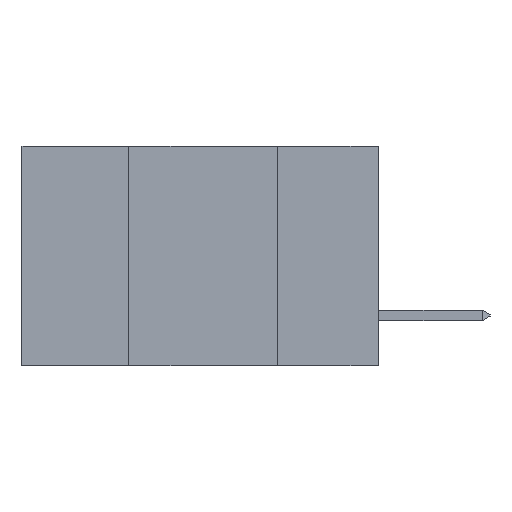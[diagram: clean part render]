
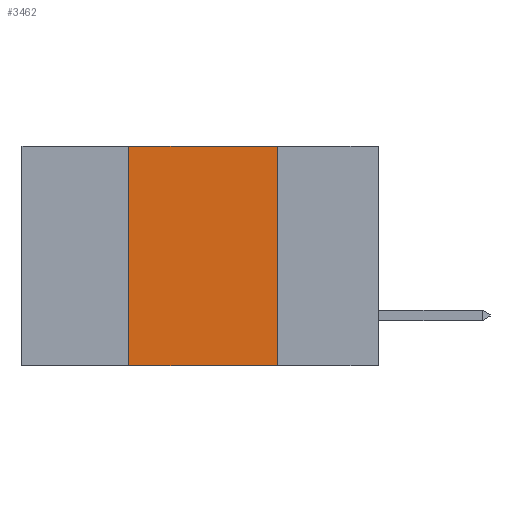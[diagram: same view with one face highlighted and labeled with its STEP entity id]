
A CAD part, left-side view. The second image highlights one B-rep face of the part: STEP entity #3462.
In plain terms, the highlighted planar face has unit normal (-1, 0, 0).
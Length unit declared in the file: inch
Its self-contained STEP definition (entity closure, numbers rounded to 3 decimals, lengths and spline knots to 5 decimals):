
#441 = LINE ( 'NONE', #831, #7234 ) ;
#478 = VERTEX_POINT ( 'NONE', #2760 ) ;
#831 = CARTESIAN_POINT ( 'NONE',  ( 0., 0.6, -0.37 ) ) ;
#945 = LINE ( 'NONE', #14482, #8116 ) ;
#1266 = VECTOR ( 'NONE', #4823, 39.37008 ) ;
#1758 = VECTOR ( 'NONE', #12450, 39.37008 ) ;
#2201 = CARTESIAN_POINT ( 'NONE',  ( 0., 0.42, -0.37 ) ) ;
#2386 = EDGE_CURVE ( 'NONE', #11320, #3335, #945, .T. ) ;
#2760 = CARTESIAN_POINT ( 'NONE',  ( 0., 0.17, -0.37 ) ) ;
#3335 = VERTEX_POINT ( 'NONE', #6868 ) ;
#3462 = ADVANCED_FACE ( 'NONE', ( #12043 ), #9267, .F. ) ;
#3794 = VERTEX_POINT ( 'NONE', #2201 ) ;
#4823 = DIRECTION ( 'NONE',  ( 0., 0., 1. ) ) ;
#6344 = ORIENTED_EDGE ( 'NONE', *, *, #2386, .F. ) ;
#6868 = CARTESIAN_POINT ( 'NONE',  ( 0., 0.17, 0. ) ) ;
#7234 = VECTOR ( 'NONE', #13904, 39.37008 ) ;
#8116 = VECTOR ( 'NONE', #15686, 39.37008 ) ;
#8191 = AXIS2_PLACEMENT_3D ( 'NONE', #12550, #12734, #11760 ) ;
#8666 = CARTESIAN_POINT ( 'NONE',  ( 0., 0.17, 0. ) ) ;
#9227 = LINE ( 'NONE', #8666, #1758 ) ;
#9267 = PLANE ( 'NONE',  #8191 ) ;
#10671 = EDGE_LOOP ( 'NONE', ( #13750, #6344, #16018, #13999 ) ) ;
#10737 = EDGE_CURVE ( 'NONE', #3335, #478, #9227, .T. ) ;
#10843 = EDGE_CURVE ( 'NONE', #3794, #478, #441, .T. ) ;
#11320 = VERTEX_POINT ( 'NONE', #14711 ) ;
#11691 = EDGE_CURVE ( 'NONE', #3794, #11320, #14331, .T. ) ;
#11760 = DIRECTION ( 'NONE',  ( 0., 0., -1. ) ) ;
#12043 = FACE_OUTER_BOUND ( 'NONE', #10671, .T. ) ;
#12450 = DIRECTION ( 'NONE',  ( 0., 0., -1. ) ) ;
#12550 = CARTESIAN_POINT ( 'NONE',  ( 0., 0.6, 0. ) ) ;
#12560 = CARTESIAN_POINT ( 'NONE',  ( 0., 0.42, 0. ) ) ;
#12734 = DIRECTION ( 'NONE',  ( 1., 0., 0. ) ) ;
#13750 = ORIENTED_EDGE ( 'NONE', *, *, #10737, .F. ) ;
#13904 = DIRECTION ( 'NONE',  ( 0., -1., 0. ) ) ;
#13999 = ORIENTED_EDGE ( 'NONE', *, *, #10843, .T. ) ;
#14331 = LINE ( 'NONE', #12560, #1266 ) ;
#14482 = CARTESIAN_POINT ( 'NONE',  ( 0., 0.6, 0. ) ) ;
#14711 = CARTESIAN_POINT ( 'NONE',  ( 0., 0.42, 0. ) ) ;
#15686 = DIRECTION ( 'NONE',  ( 0., -1., 0. ) ) ;
#16018 = ORIENTED_EDGE ( 'NONE', *, *, #11691, .F. ) ;
